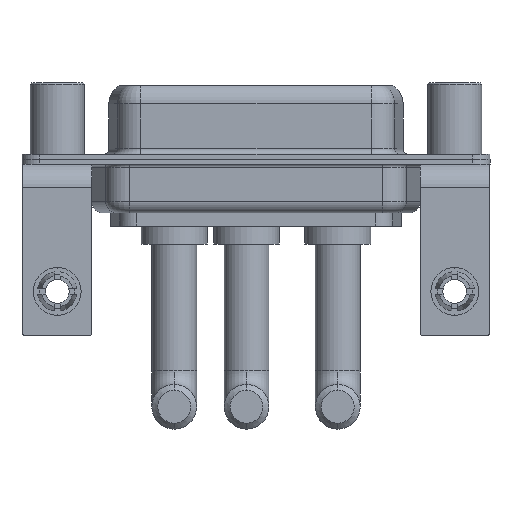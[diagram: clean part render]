
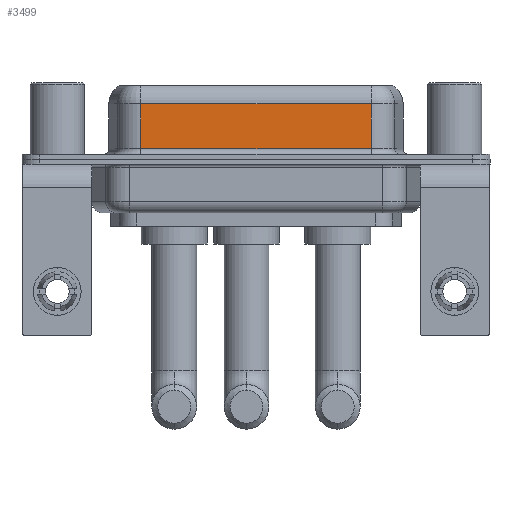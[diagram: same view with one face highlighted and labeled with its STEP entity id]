
A CAD part, front view. The second image highlights one B-rep face of the part: STEP entity #3499.
In plain terms, the highlighted planar face has unit normal (0, -1, 0).
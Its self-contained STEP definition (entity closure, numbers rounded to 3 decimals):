
#193 = VERTEX_POINT ( 'NONE', #10353 ) ;
#1092 = PLANE ( 'NONE',  #11990 ) ;
#1094 = LINE ( 'NONE', #1455, #10185 ) ;
#1425 = CARTESIAN_POINT ( 'NONE',  ( 7.013, -3.95, 4.65 ) ) ;
#1455 = CARTESIAN_POINT ( 'NONE',  ( 26.287, -3.95, 0.9 ) ) ;
#1936 = EDGE_CURVE ( 'NONE', #193, #4160, #13535, .T. ) ;
#2194 = ORIENTED_EDGE ( 'NONE', *, *, #1936, .F. ) ;
#2557 = CARTESIAN_POINT ( 'NONE',  ( 26.287, -3.95, 4.65 ) ) ;
#3144 = VECTOR ( 'NONE', #3271, 1000. ) ;
#3271 = DIRECTION ( 'NONE',  ( 0., 0., -1. ) ) ;
#3499 = ADVANCED_FACE ( 'NONE', ( #3727 ), #1092, .F. ) ;
#3727 = FACE_OUTER_BOUND ( 'NONE', #13849, .T. ) ;
#4160 = VERTEX_POINT ( 'NONE', #6865 ) ;
#4898 = EDGE_CURVE ( 'NONE', #193, #10371, #7554, .T. ) ;
#5321 = DIRECTION ( 'NONE',  ( 0., 0., 1. ) ) ;
#5516 = CARTESIAN_POINT ( 'NONE',  ( 26.287, -3.95, 6.4 ) ) ;
#5892 = CARTESIAN_POINT ( 'NONE',  ( 7.013, -3.95, 0.9 ) ) ;
#6799 = DIRECTION ( 'NONE',  ( 1., 0., 0. ) ) ;
#6865 = CARTESIAN_POINT ( 'NONE',  ( 26.287, -3.95, 0.9 ) ) ;
#6982 = DIRECTION ( 'NONE',  ( 0., 0., -1. ) ) ;
#7282 = VECTOR ( 'NONE', #9123, 1000. ) ;
#7554 = LINE ( 'NONE', #2557, #7282 ) ;
#7801 = VECTOR ( 'NONE', #6982, 1000. ) ;
#8980 = DIRECTION ( 'NONE',  ( 0., 1., 0. ) ) ;
#9073 = CARTESIAN_POINT ( 'NONE',  ( 26.287, -3.95, 6.4 ) ) ;
#9123 = DIRECTION ( 'NONE',  ( -1., 0., 0. ) ) ;
#9936 = LINE ( 'NONE', #15259, #3144 ) ;
#10185 = VECTOR ( 'NONE', #6799, 1000. ) ;
#10353 = CARTESIAN_POINT ( 'NONE',  ( 26.287, -3.95, 4.65 ) ) ;
#10371 = VERTEX_POINT ( 'NONE', #1425 ) ;
#11562 = ORIENTED_EDGE ( 'NONE', *, *, #4898, .T. ) ;
#11895 = VERTEX_POINT ( 'NONE', #5892 ) ;
#11990 = AXIS2_PLACEMENT_3D ( 'NONE', #9073, #8980, #5321 ) ;
#12521 = ORIENTED_EDGE ( 'NONE', *, *, #14473, .T. ) ;
#13445 = EDGE_CURVE ( 'NONE', #10371, #11895, #9936, .T. ) ;
#13535 = LINE ( 'NONE', #5516, #7801 ) ;
#13849 = EDGE_LOOP ( 'NONE', ( #2194, #11562, #17116, #12521 ) ) ;
#14473 = EDGE_CURVE ( 'NONE', #11895, #4160, #1094, .T. ) ;
#15259 = CARTESIAN_POINT ( 'NONE',  ( 7.013, -3.95, 6.4 ) ) ;
#17116 = ORIENTED_EDGE ( 'NONE', *, *, #13445, .T. ) ;
